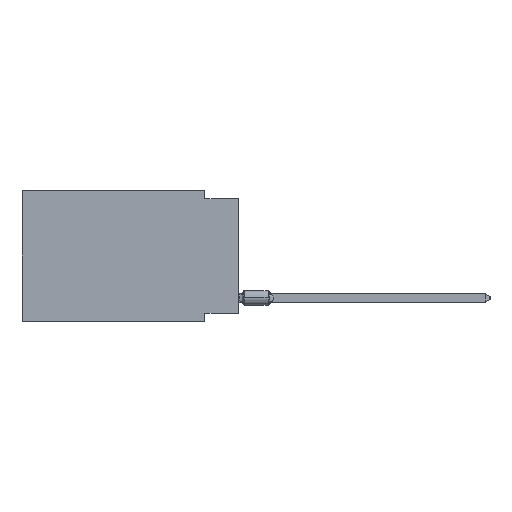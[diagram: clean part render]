
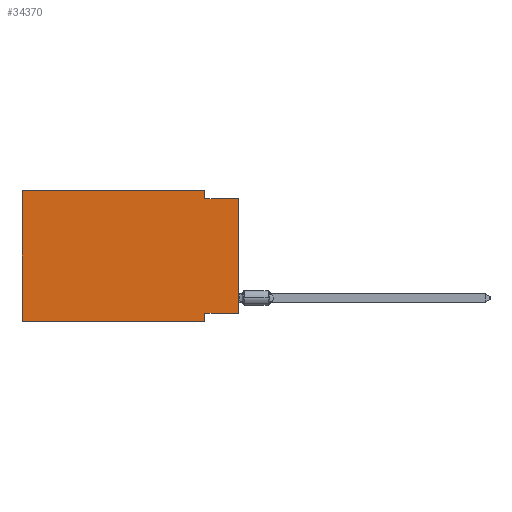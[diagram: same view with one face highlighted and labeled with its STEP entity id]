
A CAD part, left-side view. The second image highlights one B-rep face of the part: STEP entity #34370.
In plain terms, the highlighted planar face has unit normal (-1, 0, 0).
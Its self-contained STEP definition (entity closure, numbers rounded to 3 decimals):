
#93 = LINE ( 'NONE', #10291, #22298 ) ;
#2213 = CARTESIAN_POINT ( 'NONE',  ( 0., 16.383, 0. ) ) ;
#2829 = LINE ( 'NONE', #31715, #12347 ) ;
#2962 = EDGE_CURVE ( 'NONE', #40517, #39149, #93, .T. ) ;
#3556 = DIRECTION ( 'NONE',  ( 0., 0., 1. ) ) ;
#3833 = EDGE_CURVE ( 'NONE', #19976, #10180, #7743, .T. ) ;
#4530 = VERTEX_POINT ( 'NONE', #42423 ) ;
#5518 = ORIENTED_EDGE ( 'NONE', *, *, #3833, .F. ) ;
#6060 = CARTESIAN_POINT ( 'NONE',  ( 0., 2.54, -9.271 ) ) ;
#6794 = LINE ( 'NONE', #20040, #29236 ) ;
#7264 = CARTESIAN_POINT ( 'NONE',  ( 0., 16.383, 0. ) ) ;
#7305 = ORIENTED_EDGE ( 'NONE', *, *, #20143, .F. ) ;
#7743 = LINE ( 'NONE', #15099, #13750 ) ;
#9249 = CARTESIAN_POINT ( 'NONE',  ( 0., 0., -0.635 ) ) ;
#9260 = VECTOR ( 'NONE', #15455, 1000. ) ;
#10082 = PLANE ( 'NONE',  #36416 ) ;
#10180 = VERTEX_POINT ( 'NONE', #20967 ) ;
#10291 = CARTESIAN_POINT ( 'NONE',  ( 0., 0., 0. ) ) ;
#10371 = EDGE_CURVE ( 'NONE', #40517, #40044, #6794, .T. ) ;
#11716 = EDGE_CURVE ( 'NONE', #15463, #39149, #11770, .T. ) ;
#11770 = LINE ( 'NONE', #18293, #13277 ) ;
#12347 = VECTOR ( 'NONE', #41704, 1000. ) ;
#13277 = VECTOR ( 'NONE', #25013, 1000. ) ;
#13750 = VECTOR ( 'NONE', #38105, 1000. ) ;
#13787 = CARTESIAN_POINT ( 'NONE',  ( 0., 16.383, 0. ) ) ;
#14843 = CARTESIAN_POINT ( 'NONE',  ( 0., 2.54, -9.906 ) ) ;
#15099 = CARTESIAN_POINT ( 'NONE',  ( 0., 16.383, 0. ) ) ;
#15455 = DIRECTION ( 'NONE',  ( 0., 0., 1. ) ) ;
#15463 = VERTEX_POINT ( 'NONE', #22749 ) ;
#17188 = EDGE_CURVE ( 'NONE', #10180, #15463, #2829, .T. ) ;
#17908 = LINE ( 'NONE', #14843, #35841 ) ;
#18293 = CARTESIAN_POINT ( 'NONE',  ( 0., 0., -0.635 ) ) ;
#19310 = ORIENTED_EDGE ( 'NONE', *, *, #17188, .F. ) ;
#19861 = DIRECTION ( 'NONE',  ( 0., -1., 0. ) ) ;
#19976 = VERTEX_POINT ( 'NONE', #7264 ) ;
#20040 = CARTESIAN_POINT ( 'NONE',  ( 0., 0., -9.271 ) ) ;
#20143 = EDGE_CURVE ( 'NONE', #40044, #27294, #17908, .T. ) ;
#20292 = ORIENTED_EDGE ( 'NONE', *, *, #34383, .T. ) ;
#20967 = CARTESIAN_POINT ( 'NONE',  ( 0., 2.54, 0. ) ) ;
#22298 = VECTOR ( 'NONE', #3556, 1000. ) ;
#22749 = CARTESIAN_POINT ( 'NONE',  ( 0., 2.54, -0.635 ) ) ;
#22910 = CARTESIAN_POINT ( 'NONE',  ( 0., 16.383, -9.906 ) ) ;
#23120 = DIRECTION ( 'NONE',  ( 1., 0., 0. ) ) ;
#23264 = VECTOR ( 'NONE', #19861, 1000. ) ;
#23566 = LINE ( 'NONE', #22910, #23264 ) ;
#24664 = ORIENTED_EDGE ( 'NONE', *, *, #10371, .F. ) ;
#25013 = DIRECTION ( 'NONE',  ( 0., -1., 0. ) ) ;
#25514 = EDGE_CURVE ( 'NONE', #4530, #19976, #35227, .T. ) ;
#27061 = CARTESIAN_POINT ( 'NONE',  ( 0., 0., -9.271 ) ) ;
#27184 = DIRECTION ( 'NONE',  ( 0., 1., 0. ) ) ;
#27294 = VERTEX_POINT ( 'NONE', #34831 ) ;
#28066 = DIRECTION ( 'NONE',  ( 0., 0., -1. ) ) ;
#29236 = VECTOR ( 'NONE', #27184, 1000. ) ;
#30688 = ORIENTED_EDGE ( 'NONE', *, *, #2962, .T. ) ;
#30968 = ORIENTED_EDGE ( 'NONE', *, *, #25514, .F. ) ;
#31715 = CARTESIAN_POINT ( 'NONE',  ( 0., 2.54, 0. ) ) ;
#32875 = DIRECTION ( 'NONE',  ( 0., 0., -1. ) ) ;
#34370 = ADVANCED_FACE ( 'NONE', ( #39607 ), #10082, .F. ) ;
#34383 = EDGE_CURVE ( 'NONE', #4530, #27294, #23566, .T. ) ;
#34831 = CARTESIAN_POINT ( 'NONE',  ( 0., 2.54, -9.906 ) ) ;
#35227 = LINE ( 'NONE', #2213, #9260 ) ;
#35605 = EDGE_LOOP ( 'NONE', ( #30688, #42869, #19310, #5518, #30968, #20292, #7305, #24664 ) ) ;
#35841 = VECTOR ( 'NONE', #28066, 1000. ) ;
#36416 = AXIS2_PLACEMENT_3D ( 'NONE', #13787, #23120, #32875 ) ;
#38105 = DIRECTION ( 'NONE',  ( 0., -1., 0. ) ) ;
#39149 = VERTEX_POINT ( 'NONE', #9249 ) ;
#39607 = FACE_OUTER_BOUND ( 'NONE', #35605, .T. ) ;
#40044 = VERTEX_POINT ( 'NONE', #6060 ) ;
#40517 = VERTEX_POINT ( 'NONE', #27061 ) ;
#41704 = DIRECTION ( 'NONE',  ( 0., 0., -1. ) ) ;
#42423 = CARTESIAN_POINT ( 'NONE',  ( 0., 16.383, -9.906 ) ) ;
#42869 = ORIENTED_EDGE ( 'NONE', *, *, #11716, .F. ) ;
